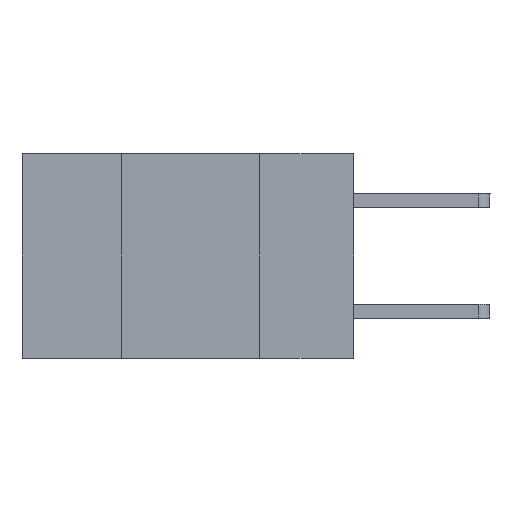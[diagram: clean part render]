
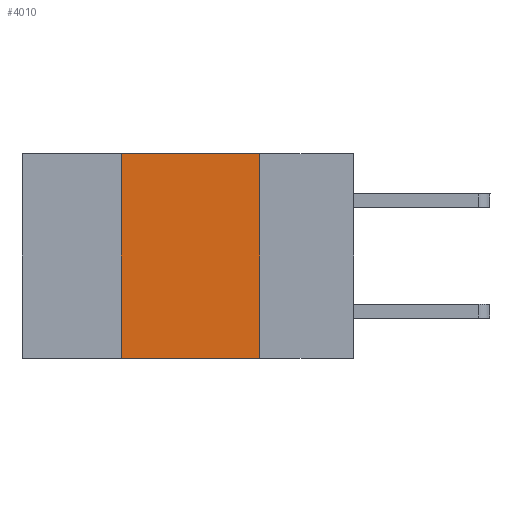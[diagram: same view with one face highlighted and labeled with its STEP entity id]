
A CAD part, left-side view. The second image highlights one B-rep face of the part: STEP entity #4010.
In plain terms, the highlighted planar face has unit normal (-1, 0, 0).
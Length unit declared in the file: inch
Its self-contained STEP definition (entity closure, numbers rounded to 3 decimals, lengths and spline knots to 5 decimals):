
#292 = EDGE_CURVE ( 'NONE', #1951, #9038, #6145, .T. ) ;
#696 = DIRECTION ( 'NONE',  ( 0., -1., 0. ) ) ;
#839 = CARTESIAN_POINT ( 'NONE',  ( 0., 0.17, -0.37 ) ) ;
#1007 = EDGE_CURVE ( 'NONE', #9038, #7580, #9533, .T. ) ;
#1763 = FACE_OUTER_BOUND ( 'NONE', #9114, .T. ) ;
#1946 = CARTESIAN_POINT ( 'NONE',  ( 0., 0.42, 0. ) ) ;
#1951 = VERTEX_POINT ( 'NONE', #6608 ) ;
#2901 = ORIENTED_EDGE ( 'NONE', *, *, #5754, .F. ) ;
#3647 = DIRECTION ( 'NONE',  ( 1., 0., 0. ) ) ;
#3675 = LINE ( 'NONE', #8614, #8972 ) ;
#3677 = DIRECTION ( 'NONE',  ( 0., 0., -1. ) ) ;
#3802 = PLANE ( 'NONE',  #8293 ) ;
#4010 = ADVANCED_FACE ( 'NONE', ( #1763 ), #3802, .F. ) ;
#4035 = VERTEX_POINT ( 'NONE', #839 ) ;
#4299 = VECTOR ( 'NONE', #696, 39.37008 ) ;
#4383 = CARTESIAN_POINT ( 'NONE',  ( 0., 0.6, 0. ) ) ;
#4944 = EDGE_CURVE ( 'NONE', #1951, #4035, #8883, .T. ) ;
#4952 = CARTESIAN_POINT ( 'NONE',  ( 0., 0.6, 0. ) ) ;
#5384 = ORIENTED_EDGE ( 'NONE', *, *, #292, .F. ) ;
#5472 = CARTESIAN_POINT ( 'NONE',  ( 0., 0.42, 0. ) ) ;
#5754 = EDGE_CURVE ( 'NONE', #7580, #4035, #3675, .T. ) ;
#6060 = CARTESIAN_POINT ( 'NONE',  ( 0., 0.6, -0.37 ) ) ;
#6145 = LINE ( 'NONE', #5472, #9538 ) ;
#6482 = DIRECTION ( 'NONE',  ( 0., -1., 0. ) ) ;
#6608 = CARTESIAN_POINT ( 'NONE',  ( 0., 0.42, -0.37 ) ) ;
#7580 = VERTEX_POINT ( 'NONE', #8163 ) ;
#8163 = CARTESIAN_POINT ( 'NONE',  ( 0., 0.17, 0. ) ) ;
#8293 = AXIS2_PLACEMENT_3D ( 'NONE', #4383, #3647, #3677 ) ;
#8614 = CARTESIAN_POINT ( 'NONE',  ( 0., 0.17, 0. ) ) ;
#8632 = DIRECTION ( 'NONE',  ( 0., 0., -1. ) ) ;
#8695 = VECTOR ( 'NONE', #6482, 39.37008 ) ;
#8883 = LINE ( 'NONE', #6060, #8695 ) ;
#8972 = VECTOR ( 'NONE', #8632, 39.37008 ) ;
#9038 = VERTEX_POINT ( 'NONE', #1946 ) ;
#9114 = EDGE_LOOP ( 'NONE', ( #2901, #9348, #5384, #9456 ) ) ;
#9348 = ORIENTED_EDGE ( 'NONE', *, *, #1007, .F. ) ;
#9456 = ORIENTED_EDGE ( 'NONE', *, *, #4944, .T. ) ;
#9459 = DIRECTION ( 'NONE',  ( 0., 0., 1. ) ) ;
#9533 = LINE ( 'NONE', #4952, #4299 ) ;
#9538 = VECTOR ( 'NONE', #9459, 39.37008 ) ;
